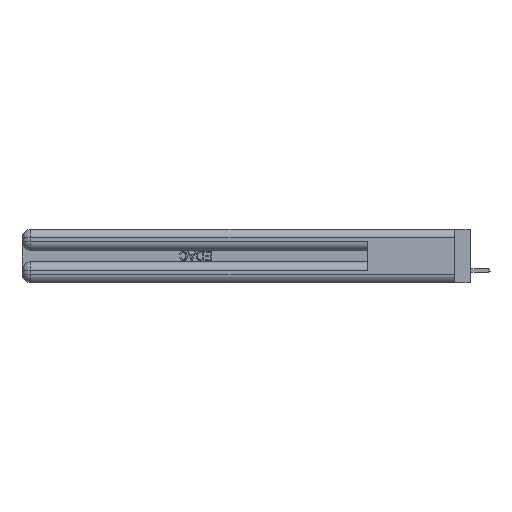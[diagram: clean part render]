
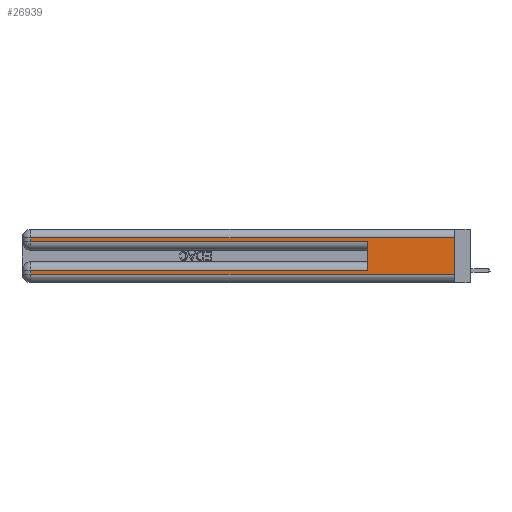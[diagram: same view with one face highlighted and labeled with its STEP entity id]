
A CAD part, left-side view. The second image highlights one B-rep face of the part: STEP entity #26939.
In plain terms, the highlighted planar face has unit normal (-1, 0, 0).
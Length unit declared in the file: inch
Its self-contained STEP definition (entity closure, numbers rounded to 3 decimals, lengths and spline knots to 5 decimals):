
#104 = DIRECTION ( 'NONE',  ( 1., 0., 0. ) ) ;
#393 = EDGE_CURVE ( 'NONE', #51241, #42271, #36424, .T. ) ;
#1101 = CARTESIAN_POINT ( 'NONE',  ( 0., 2.94, 0.37 ) ) ;
#1669 = DIRECTION ( 'NONE',  ( 0., 0., -1. ) ) ;
#2716 = LINE ( 'NONE', #46575, #47041 ) ;
#6018 = EDGE_CURVE ( 'NONE', #30148, #51241, #2716, .T. ) ;
#7620 = VECTOR ( 'NONE', #1669, 39.37008 ) ;
#7640 = LINE ( 'NONE', #43820, #51832 ) ;
#7711 = VERTEX_POINT ( 'NONE', #46598 ) ;
#8280 = DIRECTION ( 'NONE',  ( 0., 1., 0. ) ) ;
#10649 = ORIENTED_EDGE ( 'NONE', *, *, #46014, .F. ) ;
#11217 = EDGE_CURVE ( 'NONE', #23431, #42271, #16380, .T. ) ;
#11465 = EDGE_CURVE ( 'NONE', #7711, #33010, #41124, .T. ) ;
#11549 = FACE_OUTER_BOUND ( 'NONE', #17809, .T. ) ;
#12561 = CARTESIAN_POINT ( 'NONE',  ( 0., 0., 0.085 ) ) ;
#13224 = CARTESIAN_POINT ( 'NONE',  ( 0., 0.6, 0.085 ) ) ;
#13806 = CARTESIAN_POINT ( 'NONE',  ( 0., 2.94, 0.085 ) ) ;
#14188 = ORIENTED_EDGE ( 'NONE', *, *, #26090, .T. ) ;
#15029 = CARTESIAN_POINT ( 'NONE',  ( 0., 0., 0.06 ) ) ;
#15851 = CARTESIAN_POINT ( 'NONE',  ( 0., 2.94, 0.285 ) ) ;
#16100 = VECTOR ( 'NONE', #8280, 39.37008 ) ;
#16380 = LINE ( 'NONE', #31718, #17013 ) ;
#16690 = CARTESIAN_POINT ( 'NONE',  ( 0., 0., 0.285 ) ) ;
#16777 = VERTEX_POINT ( 'NONE', #13224 ) ;
#17013 = VECTOR ( 'NONE', #37535, 39.37008 ) ;
#17597 = VECTOR ( 'NONE', #20458, 39.37008 ) ;
#17809 = EDGE_LOOP ( 'NONE', ( #39400, #14188, #21870, #33720, #10649, #51135, #50106, #49295 ) ) ;
#19328 = CARTESIAN_POINT ( 'NONE',  ( 0., 0., 0.31 ) ) ;
#20458 = DIRECTION ( 'NONE',  ( 0., -1., 0. ) ) ;
#20991 = PLANE ( 'NONE',  #46258 ) ;
#21870 = ORIENTED_EDGE ( 'NONE', *, *, #11465, .T. ) ;
#23431 = VERTEX_POINT ( 'NONE', #19328 ) ;
#23453 = VERTEX_POINT ( 'NONE', #55064 ) ;
#26090 = EDGE_CURVE ( 'NONE', #23431, #7711, #7640, .T. ) ;
#26939 = ADVANCED_FACE ( 'NONE', ( #11549 ), #20991, .F. ) ;
#29086 = VECTOR ( 'NONE', #39944, 39.37008 ) ;
#29124 = DIRECTION ( 'NONE',  ( 0., 0., -1. ) ) ;
#30148 = VERTEX_POINT ( 'NONE', #13806 ) ;
#31718 = CARTESIAN_POINT ( 'NONE',  ( 0., 0., 0.37 ) ) ;
#33010 = VERTEX_POINT ( 'NONE', #15851 ) ;
#33720 = ORIENTED_EDGE ( 'NONE', *, *, #52107, .T. ) ;
#34072 = CARTESIAN_POINT ( 'NONE',  ( 0., 0., 0.37 ) ) ;
#36336 = DIRECTION ( 'NONE',  ( 0., 1., 0. ) ) ;
#36424 = LINE ( 'NONE', #43657, #54578 ) ;
#37005 = LINE ( 'NONE', #16690, #17597 ) ;
#37535 = DIRECTION ( 'NONE',  ( 0., 0., -1. ) ) ;
#39400 = ORIENTED_EDGE ( 'NONE', *, *, #11217, .F. ) ;
#39944 = DIRECTION ( 'NONE',  ( 0., 0., 1. ) ) ;
#40777 = EDGE_CURVE ( 'NONE', #16777, #30148, #46946, .T. ) ;
#41124 = LINE ( 'NONE', #1101, #7620 ) ;
#42271 = VERTEX_POINT ( 'NONE', #15029 ) ;
#43657 = CARTESIAN_POINT ( 'NONE',  ( 0., 0., 0.06 ) ) ;
#43820 = CARTESIAN_POINT ( 'NONE',  ( 0., 0., 0.31 ) ) ;
#44611 = CARTESIAN_POINT ( 'NONE',  ( 0., 2.94, 0.06 ) ) ;
#46014 = EDGE_CURVE ( 'NONE', #16777, #23453, #51210, .T. ) ;
#46258 = AXIS2_PLACEMENT_3D ( 'NONE', #34072, #104, #47328 ) ;
#46575 = CARTESIAN_POINT ( 'NONE',  ( 0., 2.94, 0.37 ) ) ;
#46598 = CARTESIAN_POINT ( 'NONE',  ( 0., 2.94, 0.31 ) ) ;
#46946 = LINE ( 'NONE', #12561, #16100 ) ;
#47041 = VECTOR ( 'NONE', #29124, 39.37008 ) ;
#47328 = DIRECTION ( 'NONE',  ( 0., 0., -1. ) ) ;
#49295 = ORIENTED_EDGE ( 'NONE', *, *, #393, .T. ) ;
#50106 = ORIENTED_EDGE ( 'NONE', *, *, #6018, .T. ) ;
#51135 = ORIENTED_EDGE ( 'NONE', *, *, #40777, .T. ) ;
#51210 = LINE ( 'NONE', #53224, #29086 ) ;
#51241 = VERTEX_POINT ( 'NONE', #44611 ) ;
#51832 = VECTOR ( 'NONE', #36336, 39.37008 ) ;
#52107 = EDGE_CURVE ( 'NONE', #33010, #23453, #37005, .T. ) ;
#52237 = DIRECTION ( 'NONE',  ( 0., -1., 0. ) ) ;
#53224 = CARTESIAN_POINT ( 'NONE',  ( 0., 0.6, 0.145 ) ) ;
#54578 = VECTOR ( 'NONE', #52237, 39.37008 ) ;
#55064 = CARTESIAN_POINT ( 'NONE',  ( 0., 0.6, 0.285 ) ) ;
